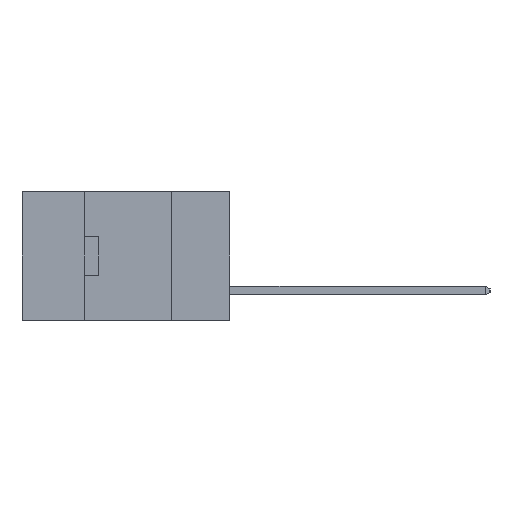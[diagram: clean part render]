
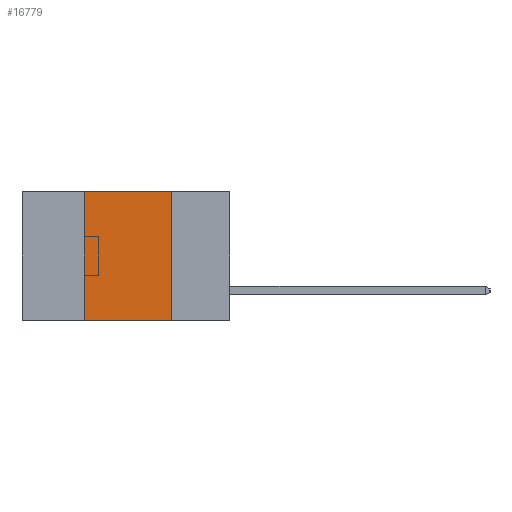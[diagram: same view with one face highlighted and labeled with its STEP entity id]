
A CAD part, left-side view. The second image highlights one B-rep face of the part: STEP entity #16779.
In plain terms, the highlighted planar face has unit normal (-1, 0, 0).
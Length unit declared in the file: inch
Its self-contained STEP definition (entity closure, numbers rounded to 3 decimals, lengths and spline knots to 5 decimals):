
#479 = ORIENTED_EDGE ( 'NONE', *, *, #8588, .F. ) ;
#767 = ORIENTED_EDGE ( 'NONE', *, *, #19716, .F. ) ;
#893 = DIRECTION ( 'NONE',  ( 0., -1., 0. ) ) ;
#1253 = VERTEX_POINT ( 'NONE', #13317 ) ;
#1881 = VECTOR ( 'NONE', #7768, 39.37008 ) ;
#2184 = VECTOR ( 'NONE', #10935, 39.37008 ) ;
#2644 = DIRECTION ( 'NONE',  ( 0., -1., 0. ) ) ;
#3793 = PLANE ( 'NONE',  #14365 ) ;
#4010 = VERTEX_POINT ( 'NONE', #20441 ) ;
#5176 = ORIENTED_EDGE ( 'NONE', *, *, #11833, .T. ) ;
#5781 = CARTESIAN_POINT ( 'NONE',  ( 0., 0.42, -0.37 ) ) ;
#7768 = DIRECTION ( 'NONE',  ( 0., 0., 1. ) ) ;
#8588 = EDGE_CURVE ( 'NONE', #13774, #4010, #23911, .T. ) ;
#9363 = VECTOR ( 'NONE', #2644, 39.37008 ) ;
#10030 = DIRECTION ( 'NONE',  ( 0., 0., -1. ) ) ;
#10935 = DIRECTION ( 'NONE',  ( 0., 0., -1. ) ) ;
#11004 = CARTESIAN_POINT ( 'NONE',  ( 0., 0.17, -0.37 ) ) ;
#11070 = CARTESIAN_POINT ( 'NONE',  ( 0., 0.17, 0. ) ) ;
#11833 = EDGE_CURVE ( 'NONE', #18949, #4010, #16714, .T. ) ;
#12021 = CARTESIAN_POINT ( 'NONE',  ( 0., 0.6, 0. ) ) ;
#12481 = CARTESIAN_POINT ( 'NONE',  ( 0., 0.42, -0.37 ) ) ;
#12993 = CARTESIAN_POINT ( 'NONE',  ( 0., 0.6, 0. ) ) ;
#13317 = CARTESIAN_POINT ( 'NONE',  ( 0., 0.42, 0. ) ) ;
#13607 = LINE ( 'NONE', #5781, #1881 ) ;
#13774 = VERTEX_POINT ( 'NONE', #11070 ) ;
#14365 = AXIS2_PLACEMENT_3D ( 'NONE', #12021, #22214, #10030 ) ;
#15448 = CARTESIAN_POINT ( 'NONE',  ( 0., 0.6, -0.37 ) ) ;
#16714 = LINE ( 'NONE', #15448, #21411 ) ;
#16779 = ADVANCED_FACE ( 'NONE', ( #20392 ), #3793, .F. ) ;
#17613 = ORIENTED_EDGE ( 'NONE', *, *, #24220, .F. ) ;
#18573 = EDGE_LOOP ( 'NONE', ( #479, #767, #17613, #5176 ) ) ;
#18949 = VERTEX_POINT ( 'NONE', #12481 ) ;
#19566 = LINE ( 'NONE', #12993, #9363 ) ;
#19716 = EDGE_CURVE ( 'NONE', #1253, #13774, #19566, .T. ) ;
#20392 = FACE_OUTER_BOUND ( 'NONE', #18573, .T. ) ;
#20441 = CARTESIAN_POINT ( 'NONE',  ( 0., 0.17, -0.37 ) ) ;
#21411 = VECTOR ( 'NONE', #893, 39.37008 ) ;
#22214 = DIRECTION ( 'NONE',  ( 1., 0., 0. ) ) ;
#23911 = LINE ( 'NONE', #11004, #2184 ) ;
#24220 = EDGE_CURVE ( 'NONE', #18949, #1253, #13607, .T. ) ;
